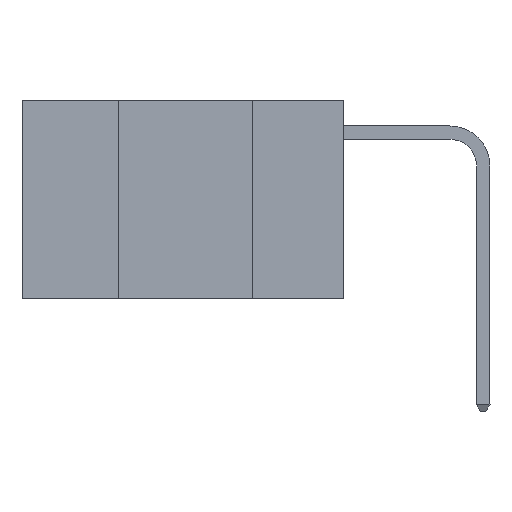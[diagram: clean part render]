
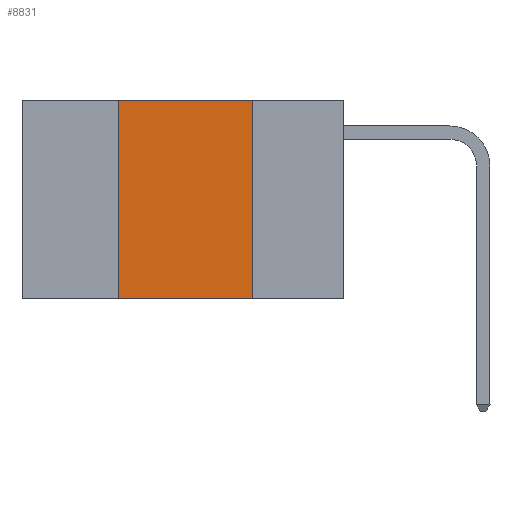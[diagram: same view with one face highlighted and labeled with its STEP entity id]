
A CAD part, left-side view. The second image highlights one B-rep face of the part: STEP entity #8831.
In plain terms, the highlighted planar face has unit normal (-1, 0, 0).
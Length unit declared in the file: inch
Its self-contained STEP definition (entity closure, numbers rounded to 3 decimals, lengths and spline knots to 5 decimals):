
#16 = ORIENTED_EDGE ( 'NONE', *, *, #8894, .F. ) ;
#165 = DIRECTION ( 'NONE',  ( 0., 0., 1. ) ) ;
#184 = FACE_OUTER_BOUND ( 'NONE', #1678, .T. ) ;
#338 = DIRECTION ( 'NONE',  ( 0., -1., 0. ) ) ;
#390 = CARTESIAN_POINT ( 'NONE',  ( 0., 0.6, 0. ) ) ;
#396 = VERTEX_POINT ( 'NONE', #2680 ) ;
#433 = VECTOR ( 'NONE', #4656, 39.37008 ) ;
#778 = ORIENTED_EDGE ( 'NONE', *, *, #2636, .F. ) ;
#865 = PLANE ( 'NONE',  #4540 ) ;
#1020 = DIRECTION ( 'NONE',  ( 0., 0., -1. ) ) ;
#1135 = CARTESIAN_POINT ( 'NONE',  ( 0., 0.42, -0.37 ) ) ;
#1678 = EDGE_LOOP ( 'NONE', ( #778, #16, #5962, #4308 ) ) ;
#2035 = EDGE_CURVE ( 'NONE', #2255, #4561, #3757, .T. ) ;
#2082 = CARTESIAN_POINT ( 'NONE',  ( 0., 0.17, -0.37 ) ) ;
#2255 = VERTEX_POINT ( 'NONE', #1135 ) ;
#2338 = CARTESIAN_POINT ( 'NONE',  ( 0., 0.6, 0. ) ) ;
#2636 = EDGE_CURVE ( 'NONE', #396, #4561, #3900, .T. ) ;
#2680 = CARTESIAN_POINT ( 'NONE',  ( 0., 0.17, 0. ) ) ;
#2715 = VECTOR ( 'NONE', #8355, 39.37008 ) ;
#3757 = LINE ( 'NONE', #6163, #2715 ) ;
#3900 = LINE ( 'NONE', #8502, #433 ) ;
#4042 = VERTEX_POINT ( 'NONE', #5726 ) ;
#4308 = ORIENTED_EDGE ( 'NONE', *, *, #2035, .T. ) ;
#4540 = AXIS2_PLACEMENT_3D ( 'NONE', #2338, #6249, #1020 ) ;
#4561 = VERTEX_POINT ( 'NONE', #2082 ) ;
#4656 = DIRECTION ( 'NONE',  ( 0., 0., -1. ) ) ;
#5535 = CARTESIAN_POINT ( 'NONE',  ( 0., 0.42, 0. ) ) ;
#5726 = CARTESIAN_POINT ( 'NONE',  ( 0., 0.42, 0. ) ) ;
#5962 = ORIENTED_EDGE ( 'NONE', *, *, #8176, .F. ) ;
#5990 = VECTOR ( 'NONE', #338, 39.37008 ) ;
#6163 = CARTESIAN_POINT ( 'NONE',  ( 0., 0.6, -0.37 ) ) ;
#6249 = DIRECTION ( 'NONE',  ( 1., 0., 0. ) ) ;
#7212 = LINE ( 'NONE', #390, #5990 ) ;
#8176 = EDGE_CURVE ( 'NONE', #2255, #4042, #9177, .T. ) ;
#8193 = VECTOR ( 'NONE', #165, 39.37008 ) ;
#8355 = DIRECTION ( 'NONE',  ( 0., -1., 0. ) ) ;
#8502 = CARTESIAN_POINT ( 'NONE',  ( 0., 0.17, 0. ) ) ;
#8831 = ADVANCED_FACE ( 'NONE', ( #184 ), #865, .F. ) ;
#8894 = EDGE_CURVE ( 'NONE', #4042, #396, #7212, .T. ) ;
#9177 = LINE ( 'NONE', #5535, #8193 ) ;
